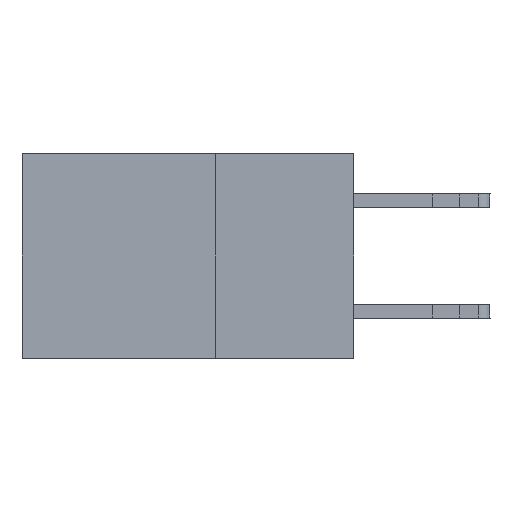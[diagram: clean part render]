
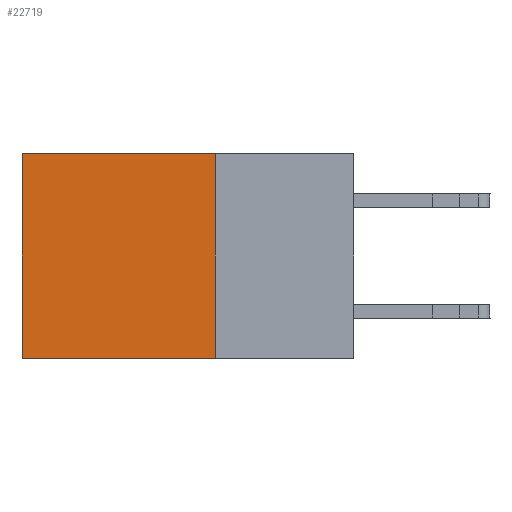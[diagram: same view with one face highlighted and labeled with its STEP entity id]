
A CAD part, left-side view. The second image highlights one B-rep face of the part: STEP entity #22719.
In plain terms, the highlighted planar face has unit normal (-1, 0, 0).
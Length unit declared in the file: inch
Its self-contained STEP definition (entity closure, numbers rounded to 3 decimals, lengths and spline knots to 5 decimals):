
#278 = ORIENTED_EDGE ( 'NONE', *, *, #18649, .F. ) ;
#468 = VECTOR ( 'NONE', #17511, 39.37008 ) ;
#549 = FACE_OUTER_BOUND ( 'NONE', #26987, .T. ) ;
#841 = DIRECTION ( 'NONE',  ( 0., 0., -1. ) ) ;
#871 = ORIENTED_EDGE ( 'NONE', *, *, #9995, .T. ) ;
#1432 = VECTOR ( 'NONE', #23635, 39.37008 ) ;
#3353 = LINE ( 'NONE', #23910, #4381 ) ;
#4381 = VECTOR ( 'NONE', #19733, 39.37008 ) ;
#4548 = CARTESIAN_POINT ( 'NONE',  ( 0.2875, 0.25, 0. ) ) ;
#5325 = CARTESIAN_POINT ( 'NONE',  ( 0.2875, 0.25, 0. ) ) ;
#9921 = VERTEX_POINT ( 'NONE', #21081 ) ;
#9995 = EDGE_CURVE ( 'NONE', #9921, #26184, #3353, .T. ) ;
#10363 = CARTESIAN_POINT ( 'NONE',  ( 0.2875, 0.25, 0. ) ) ;
#13229 = CARTESIAN_POINT ( 'NONE',  ( 0.2875, 0.25, -0.37 ) ) ;
#14140 = CARTESIAN_POINT ( 'NONE',  ( 0.2875, 0.25, 0. ) ) ;
#14537 = VECTOR ( 'NONE', #28005, 39.37008 ) ;
#15141 = EDGE_CURVE ( 'NONE', #21098, #26184, #25480, .T. ) ;
#16026 = CARTESIAN_POINT ( 'NONE',  ( 0.2875, 0.6, -0.37 ) ) ;
#16659 = LINE ( 'NONE', #5325, #1432 ) ;
#16834 = AXIS2_PLACEMENT_3D ( 'NONE', #14140, #28106, #841 ) ;
#17511 = DIRECTION ( 'NONE',  ( 0., 0., -1. ) ) ;
#18649 = EDGE_CURVE ( 'NONE', #21275, #21098, #28821, .T. ) ;
#19394 = EDGE_CURVE ( 'NONE', #21275, #9921, #16659, .T. ) ;
#19733 = DIRECTION ( 'NONE',  ( 0., 0., -1. ) ) ;
#21081 = CARTESIAN_POINT ( 'NONE',  ( 0.2875, 0.6, 0. ) ) ;
#21098 = VERTEX_POINT ( 'NONE', #13229 ) ;
#21275 = VERTEX_POINT ( 'NONE', #4548 ) ;
#22719 = ADVANCED_FACE ( 'NONE', ( #549 ), #23046, .F. ) ;
#22737 = ORIENTED_EDGE ( 'NONE', *, *, #19394, .T. ) ;
#23046 = PLANE ( 'NONE',  #16834 ) ;
#23537 = CARTESIAN_POINT ( 'NONE',  ( 0.2875, 0.25, -0.37 ) ) ;
#23635 = DIRECTION ( 'NONE',  ( 0., 1., 0. ) ) ;
#23910 = CARTESIAN_POINT ( 'NONE',  ( 0.2875, 0.6, 0. ) ) ;
#24314 = ORIENTED_EDGE ( 'NONE', *, *, #15141, .F. ) ;
#25480 = LINE ( 'NONE', #23537, #14537 ) ;
#26184 = VERTEX_POINT ( 'NONE', #16026 ) ;
#26987 = EDGE_LOOP ( 'NONE', ( #871, #24314, #278, #22737 ) ) ;
#28005 = DIRECTION ( 'NONE',  ( 0., 1., 0. ) ) ;
#28106 = DIRECTION ( 'NONE',  ( 1., 0., 0. ) ) ;
#28821 = LINE ( 'NONE', #10363, #468 ) ;
